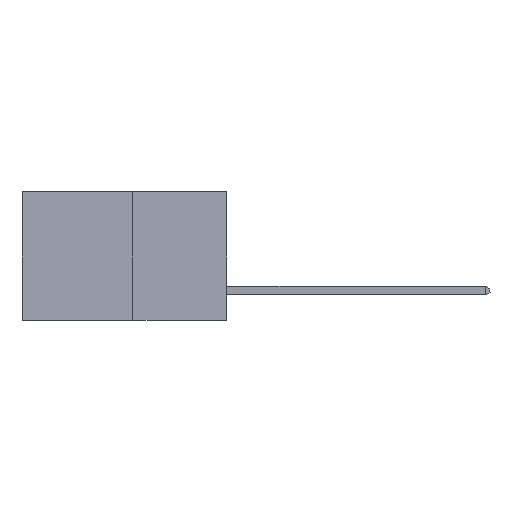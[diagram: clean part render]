
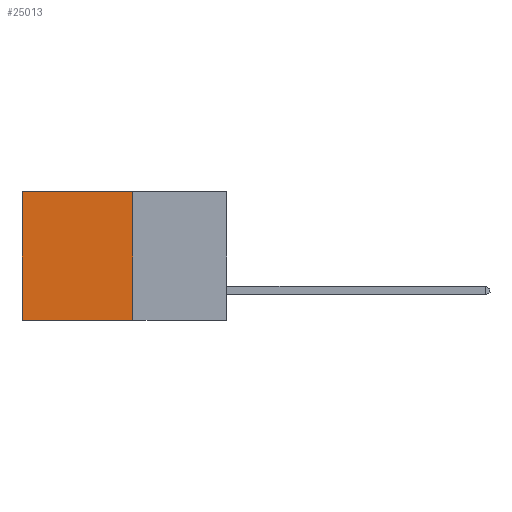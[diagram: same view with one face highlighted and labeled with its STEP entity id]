
A CAD part, left-side view. The second image highlights one B-rep face of the part: STEP entity #25013.
In plain terms, the highlighted planar face has unit normal (-1, 0, 0).
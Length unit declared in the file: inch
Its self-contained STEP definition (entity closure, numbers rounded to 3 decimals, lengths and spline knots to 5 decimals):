
#564 = AXIS2_PLACEMENT_3D ( 'NONE', #11404, #25815, #13481 ) ;
#2202 = LINE ( 'NONE', #21402, #7197 ) ;
#2467 = FACE_OUTER_BOUND ( 'NONE', #7790, .T. ) ;
#2562 = CARTESIAN_POINT ( 'NONE',  ( 0.277, 0.27, 0. ) ) ;
#2828 = VECTOR ( 'NONE', #25451, 39.37008 ) ;
#3705 = VERTEX_POINT ( 'NONE', #27043 ) ;
#3991 = VERTEX_POINT ( 'NONE', #15760 ) ;
#4568 = VERTEX_POINT ( 'NONE', #24536 ) ;
#4664 = DIRECTION ( 'NONE',  ( 0., 1., 0. ) ) ;
#5136 = EDGE_CURVE ( 'NONE', #17732, #3705, #14308, .T. ) ;
#7197 = VECTOR ( 'NONE', #4664, 39.37008 ) ;
#7790 = EDGE_LOOP ( 'NONE', ( #13184, #14286, #18548, #9423 ) ) ;
#9423 = ORIENTED_EDGE ( 'NONE', *, *, #15925, .T. ) ;
#10401 = CARTESIAN_POINT ( 'NONE',  ( 0.277, 0.59, -0.37 ) ) ;
#11404 = CARTESIAN_POINT ( 'NONE',  ( 0.277, 0.27, -0.37 ) ) ;
#12499 = DIRECTION ( 'NONE',  ( 0., 0., -1. ) ) ;
#13184 = ORIENTED_EDGE ( 'NONE', *, *, #18649, .T. ) ;
#13481 = DIRECTION ( 'NONE',  ( 0., 0., -1. ) ) ;
#13643 = VECTOR ( 'NONE', #17752, 39.37008 ) ;
#14286 = ORIENTED_EDGE ( 'NONE', *, *, #24000, .F. ) ;
#14308 = LINE ( 'NONE', #17714, #13643 ) ;
#15760 = CARTESIAN_POINT ( 'NONE',  ( 0.277, 0.59, -0.37 ) ) ;
#15925 = EDGE_CURVE ( 'NONE', #17732, #4568, #25028, .T. ) ;
#17714 = CARTESIAN_POINT ( 'NONE',  ( 0.277, 0.27, -0.37 ) ) ;
#17732 = VERTEX_POINT ( 'NONE', #22813 ) ;
#17752 = DIRECTION ( 'NONE',  ( 0., 0., -1. ) ) ;
#18548 = ORIENTED_EDGE ( 'NONE', *, *, #5136, .F. ) ;
#18649 = EDGE_CURVE ( 'NONE', #4568, #3991, #21066, .T. ) ;
#21066 = LINE ( 'NONE', #10401, #24524 ) ;
#21402 = CARTESIAN_POINT ( 'NONE',  ( 0.277, 0.27, -0.37 ) ) ;
#21711 = PLANE ( 'NONE',  #564 ) ;
#22813 = CARTESIAN_POINT ( 'NONE',  ( 0.277, 0.27, 0. ) ) ;
#24000 = EDGE_CURVE ( 'NONE', #3705, #3991, #2202, .T. ) ;
#24524 = VECTOR ( 'NONE', #12499, 39.37008 ) ;
#24536 = CARTESIAN_POINT ( 'NONE',  ( 0.277, 0.59, 0. ) ) ;
#25013 = ADVANCED_FACE ( 'NONE', ( #2467 ), #21711, .F. ) ;
#25028 = LINE ( 'NONE', #2562, #2828 ) ;
#25451 = DIRECTION ( 'NONE',  ( 0., 1., 0. ) ) ;
#25815 = DIRECTION ( 'NONE',  ( 1., 0., 0. ) ) ;
#27043 = CARTESIAN_POINT ( 'NONE',  ( 0.277, 0.27, -0.37 ) ) ;
